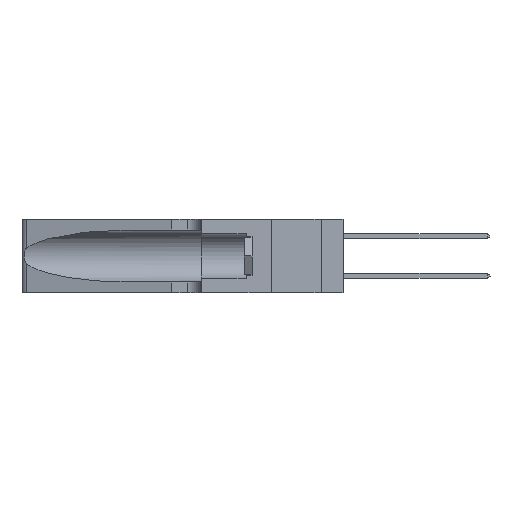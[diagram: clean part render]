
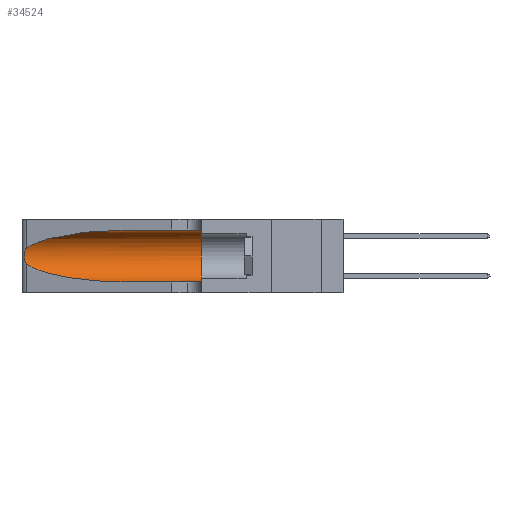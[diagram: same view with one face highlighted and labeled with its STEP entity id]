
A CAD part, left-side view. The second image highlights one B-rep face of the part: STEP entity #34524.
In plain terms, the highlighted cylindrical face has radius 3.308 mm (diameter 6.617 mm), a partial arc.
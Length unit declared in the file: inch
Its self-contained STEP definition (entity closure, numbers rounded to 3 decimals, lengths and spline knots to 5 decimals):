
#406 = CARTESIAN_POINT ( 'NONE',  ( 0.18966, 0.96281, 0.05475 ) ) ;
#648 = CARTESIAN_POINT ( 'NONE',  ( 0.1305, 0.35, 0.31525 ) ) ;
#3138 = ORIENTED_EDGE ( 'NONE', *, *, #30279, .T. ) ;
#4860 = CARTESIAN_POINT ( 'NONE',  ( 0.18966, 0.96281, 0.31525 ) ) ;
#5167 = AXIS2_PLACEMENT_3D ( 'NONE', #25544, #31297, #15200 ) ;
#5374 = CYLINDRICAL_SURFACE ( 'NONE', #5167, 0.13025 ) ;
#5965 = CARTESIAN_POINT ( 'NONE',  ( 0.25487, 1.22718, 0.14631 ) ) ;
#6001 = CARTESIAN_POINT ( 'NONE',  ( 0.25555, 1.22994, 0.2215 ) ) ;
#6120 = VERTEX_POINT ( 'NONE', #27548 ) ;
#6236 = VERTEX_POINT ( 'NONE', #40999 ) ;
#7384 = LINE ( 'NONE', #41177, #40249 ) ;
#8836 = CARTESIAN_POINT ( 'NONE',  ( 0.25639, 1.23184, 0.21858 ) ) ;
#8850 = AXIS2_PLACEMENT_3D ( 'NONE', #9675, #19149, #32293 ) ;
#9380 = CARTESIAN_POINT ( 'NONE',  ( 0.1305, 0.72297, 0.31525 ) ) ;
#9675 = CARTESIAN_POINT ( 'NONE',  ( 0.1305, 0.35, 0.185 ) ) ;
#9939 = CARTESIAN_POINT ( 'NONE',  ( 0.26018, 1.23835, 0.19895 ) ) ;
#11233 = CARTESIAN_POINT ( 'NONE',  ( 0.25555, 1.22993, 0.14849 ) ) ;
#11412 = EDGE_CURVE ( 'NONE', #31782, #18277, #21754, .T. ) ;
#11503 = CARTESIAN_POINT ( 'NONE',  ( 0.25487, 1.22718, 0.22369 ) ) ;
#13584 = EDGE_CURVE ( 'NONE', #6120, #6236, #7384, .T. ) ;
#14571 = CARTESIAN_POINT ( 'NONE',  ( 0.25487, 1.22718, 0.22369 ) ) ;
#15200 = DIRECTION ( 'NONE',  ( 0., 0., -1. ) ) ;
#15347 = CARTESIAN_POINT ( 'NONE',  ( 0.25787, 1.23484, 0.2124 ) ) ;
#15443 = ORIENTED_EDGE ( 'NONE', *, *, #37989, .F. ) ;
#15940 = DIRECTION ( 'NONE',  ( 0., -1., 0. ) ) ;
#17571 = CARTESIAN_POINT ( 'NONE',  ( 0.25856, 1.23593, 0.16098 ) ) ;
#18050 = CIRCLE ( 'NONE', #8850, 0.13025 ) ;
#18277 = VERTEX_POINT ( 'NONE', #36227 ) ;
#18574 = CARTESIAN_POINT ( 'NONE',  ( 0.25854, 1.2359, 0.20912 ) ) ;
#18988 = CARTESIAN_POINT ( 'NONE',  ( 0.26075, 1.23896, 0.19203 ) ) ;
#19149 = DIRECTION ( 'NONE',  ( 0., 1., 0. ) ) ;
#20379 = EDGE_CURVE ( 'NONE', #24611, #6236, #18050, .T. ) ;
#21754 = B_SPLINE_CURVE_WITH_KNOTS ( 'NONE', 3,
 ( #22143, #6001, #8836, #15347, #18574, #9939, #18988, #22708, #29159, #17571, #30702, #33532, #11233, #5965 ),
 .UNSPECIFIED., .F., .F.,
 ( 4, 2, 2, 2, 2, 2, 4 ),
 ( 0., 0.00027, 0.00053, 0.00107, 0.0016, 0.00187, 0.00214 ),
 .UNSPECIFIED. ) ;
#22143 = CARTESIAN_POINT ( 'NONE',  ( 0.25487, 1.22718, 0.22369 ) ) ;
#22708 = CARTESIAN_POINT ( 'NONE',  ( 0.26075, 1.23896, 0.178 ) ) ;
#22901 = CARTESIAN_POINT ( 'NONE',  ( 0.2373, 1.15595, 0.08982 ) ) ;
#24611 = VERTEX_POINT ( 'NONE', #648 ) ;
#25544 = CARTESIAN_POINT ( 'NONE',  ( 0.1305, 1.61858, 0.185 ) ) ;
#25637 = VECTOR ( 'NONE', #33976, 39.37008 ) ;
#26016 = CARTESIAN_POINT ( 'NONE',  ( 0.1305, 0.72297, 0.05475 ) ) ;
#26264 = CARTESIAN_POINT ( 'NONE',  ( 0.25487, 1.22718, 0.14631 ) ) ;
#27548 = CARTESIAN_POINT ( 'NONE',  ( 0.1305, 0.72297, 0.05475 ) ) ;
#28266 = ORIENTED_EDGE ( 'NONE', *, *, #11412, .T. ) ;
#28681 = ORIENTED_EDGE ( 'NONE', *, *, #20379, .F. ) ;
#29159 = CARTESIAN_POINT ( 'NONE',  ( 0.26017, 1.23833, 0.17102 ) ) ;
#29598 = ORIENTED_EDGE ( 'NONE', *, *, #13584, .T. ) ;
#30279 = EDGE_CURVE ( 'NONE', #18277, #6120, #30532, .T. ) ;
#30532 =( BOUNDED_CURVE ( )  B_SPLINE_CURVE ( 3, ( #26264, #22901, #406, #26016 ),
 .UNSPECIFIED., .F., .F. ) 
 B_SPLINE_CURVE_WITH_KNOTS ( ( 4, 4 ),
 ( 3.44316, 4.71239 ),
 .UNSPECIFIED. ) 
 CURVE ( )  GEOMETRIC_REPRESENTATION_ITEM ( )  RATIONAL_B_SPLINE_CURVE ( ( 1., 0.87, 0.87, 1. ) ) 
 REPRESENTATION_ITEM ( '' )  );
#30692 = CARTESIAN_POINT ( 'NONE',  ( 0.2373, 1.15595, 0.28018 ) ) ;
#30702 = CARTESIAN_POINT ( 'NONE',  ( 0.25789, 1.23486, 0.15765 ) ) ;
#30730 = CARTESIAN_POINT ( 'NONE',  ( 0.1305, 1.61858, 0.31525 ) ) ;
#31297 = DIRECTION ( 'NONE',  ( 0., -1., 0. ) ) ;
#31625 = FACE_OUTER_BOUND ( 'NONE', #38286, .T. ) ;
#31782 = VERTEX_POINT ( 'NONE', #14571 ) ;
#32293 = DIRECTION ( 'NONE',  ( 0., 0., 1. ) ) ;
#33532 = CARTESIAN_POINT ( 'NONE',  ( 0.25639, 1.23186, 0.15144 ) ) ;
#33976 = DIRECTION ( 'NONE',  ( 0., -1., 0. ) ) ;
#34479 = ORIENTED_EDGE ( 'NONE', *, *, #38505, .T. ) ;
#34524 = ADVANCED_FACE ( 'NONE', ( #31625 ), #5374, .F. ) ;
#34921 =( BOUNDED_CURVE ( )  B_SPLINE_CURVE ( 3, ( #37320, #4860, #30692, #11503 ),
 .UNSPECIFIED., .F., .F. ) 
 B_SPLINE_CURVE_WITH_KNOTS ( ( 4, 4 ),
 ( 1.5708, 2.84003 ),
 .UNSPECIFIED. ) 
 CURVE ( )  GEOMETRIC_REPRESENTATION_ITEM ( )  RATIONAL_B_SPLINE_CURVE ( ( 1., 0.87, 0.87, 1. ) ) 
 REPRESENTATION_ITEM ( '' )  );
#35187 = LINE ( 'NONE', #30730, #25637 ) ;
#36227 = CARTESIAN_POINT ( 'NONE',  ( 0.25487, 1.22718, 0.14631 ) ) ;
#37320 = CARTESIAN_POINT ( 'NONE',  ( 0.1305, 0.72297, 0.31525 ) ) ;
#37989 = EDGE_CURVE ( 'NONE', #38344, #24611, #35187, .T. ) ;
#38286 = EDGE_LOOP ( 'NONE', ( #34479, #28266, #3138, #29598, #28681, #15443 ) ) ;
#38344 = VERTEX_POINT ( 'NONE', #9380 ) ;
#38505 = EDGE_CURVE ( 'NONE', #38344, #31782, #34921, .T. ) ;
#40249 = VECTOR ( 'NONE', #15940, 39.37008 ) ;
#40999 = CARTESIAN_POINT ( 'NONE',  ( 0.1305, 0.35, 0.05475 ) ) ;
#41177 = CARTESIAN_POINT ( 'NONE',  ( 0.1305, 1.61858, 0.05475 ) ) ;
